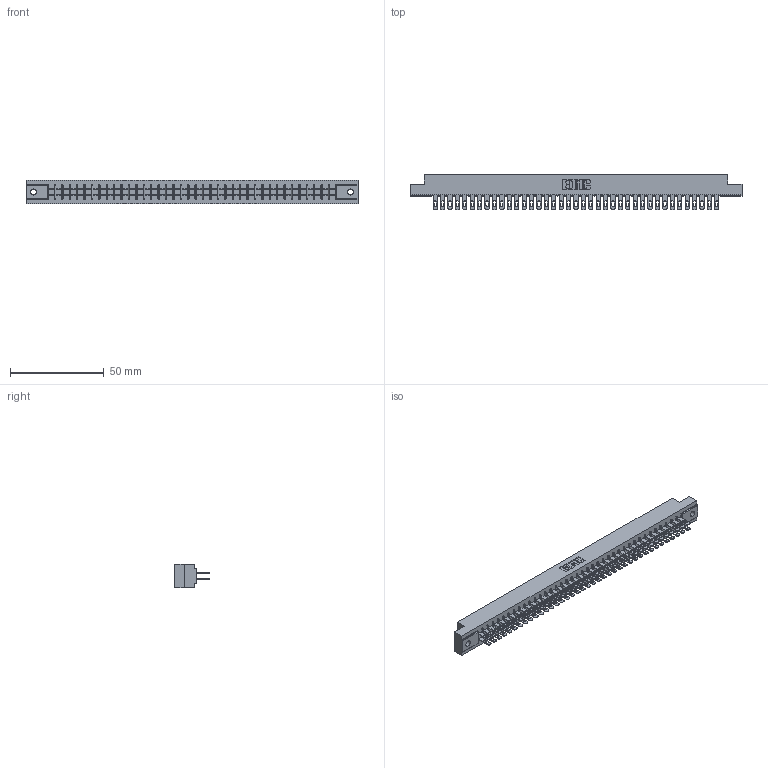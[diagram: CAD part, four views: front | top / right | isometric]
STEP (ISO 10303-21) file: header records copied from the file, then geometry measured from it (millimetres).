
FILE_DESCRIPTION (( 'STEP AP203' ), '1' );
FILE_NAME ('305-078-500-202.STEP', '2019-09-10T08:33:06', ( '' ), ( '' ), 'SwSTEP 2.0', 'SolidWorks 2016', '' );
FILE_SCHEMA (( 'CONFIG_CONTROL_DESIGN' ));
Length unit declared in the file: inch
Products named in the file (3): 305-078-500-202; 305 Part_.128 Dia; 305-290-001_500
Assembly tree (79 placements, depth 2):
  305-078-500-202
    305 Part_.128 Dia
    305-290-001_500  x78
Bounding box: 177.55 x 18.85 x 12.7 mm (x, y, z)
Volume: 18702.3 mm3; surface area: 24993.4 mm2
Topology: 79 solids, 79 shells, 4016 faces, 11509 edges, 7462 vertices
Faces by surface type: plane 2252, cylinder 1608, sphere 156
Entity records: 42616 total; most frequent: CARTESIAN_POINT 7051, ORIENTED_EDGE 6998, DIRECTION 6825, EDGE_CURVE 3499, LINE 2825, VECTOR 2825, VERTEX_POINT 2226, AXIS2_PLACEMENT_3D 2000
